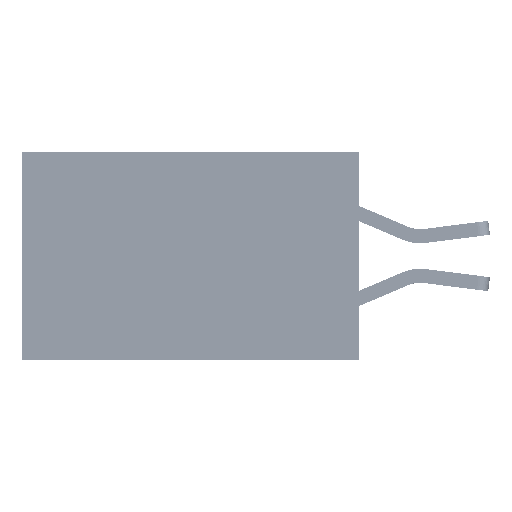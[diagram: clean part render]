
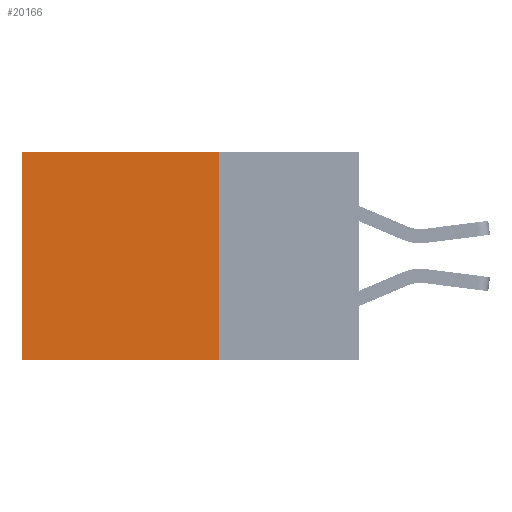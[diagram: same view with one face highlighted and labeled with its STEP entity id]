
A CAD part, left-side view. The second image highlights one B-rep face of the part: STEP entity #20166.
In plain terms, the highlighted planar face has unit normal (-1, 0, 0).
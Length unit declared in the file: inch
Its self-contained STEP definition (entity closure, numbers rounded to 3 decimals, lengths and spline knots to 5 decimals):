
#2309 = VERTEX_POINT ( 'NONE', #5757 ) ;
#3283 = LINE ( 'NONE', #34943, #49640 ) ;
#4492 = ORIENTED_EDGE ( 'NONE', *, *, #4638, .F. ) ;
#4638 = EDGE_CURVE ( 'NONE', #2309, #25689, #22918, .T. ) ;
#5257 = AXIS2_PLACEMENT_3D ( 'NONE', #21959, #42446, #38187 ) ;
#5658 = CARTESIAN_POINT ( 'NONE',  ( 0.2875, 0.25, 0. ) ) ;
#5757 = CARTESIAN_POINT ( 'NONE',  ( 0.2875, 0.25, -0.37 ) ) ;
#7684 = ORIENTED_EDGE ( 'NONE', *, *, #36085, .F. ) ;
#9734 = VERTEX_POINT ( 'NONE', #26997 ) ;
#10245 = FACE_OUTER_BOUND ( 'NONE', #40354, .T. ) ;
#11715 = ORIENTED_EDGE ( 'NONE', *, *, #41673, .T. ) ;
#14163 = LINE ( 'NONE', #5658, #38244 ) ;
#14734 = DIRECTION ( 'NONE',  ( 0., 0., -1. ) ) ;
#14960 = DIRECTION ( 'NONE',  ( 0., 1., 0. ) ) ;
#17117 = ORIENTED_EDGE ( 'NONE', *, *, #21518, .T. ) ;
#19547 = CARTESIAN_POINT ( 'NONE',  ( 0.2875, 0.6, -0.37 ) ) ;
#20166 = ADVANCED_FACE ( 'NONE', ( #10245 ), #47258, .F. ) ;
#21518 = EDGE_CURVE ( 'NONE', #37601, #9734, #42994, .T. ) ;
#21959 = CARTESIAN_POINT ( 'NONE',  ( 0.2875, 0.25, 0. ) ) ;
#22918 = LINE ( 'NONE', #31164, #44314 ) ;
#25689 = VERTEX_POINT ( 'NONE', #19547 ) ;
#26997 = CARTESIAN_POINT ( 'NONE',  ( 0.2875, 0.6, 0. ) ) ;
#27431 = VECTOR ( 'NONE', #50477, 39.37008 ) ;
#31164 = CARTESIAN_POINT ( 'NONE',  ( 0.2875, 0.25, -0.37 ) ) ;
#34202 = CARTESIAN_POINT ( 'NONE',  ( 0.2875, 0.25, 0. ) ) ;
#34943 = CARTESIAN_POINT ( 'NONE',  ( 0.2875, 0.6, 0. ) ) ;
#36085 = EDGE_CURVE ( 'NONE', #37601, #2309, #14163, .T. ) ;
#37601 = VERTEX_POINT ( 'NONE', #40502 ) ;
#38187 = DIRECTION ( 'NONE',  ( 0., 0., -1. ) ) ;
#38244 = VECTOR ( 'NONE', #50377, 39.37008 ) ;
#40354 = EDGE_LOOP ( 'NONE', ( #11715, #4492, #7684, #17117 ) ) ;
#40502 = CARTESIAN_POINT ( 'NONE',  ( 0.2875, 0.25, 0. ) ) ;
#41673 = EDGE_CURVE ( 'NONE', #9734, #25689, #3283, .T. ) ;
#42446 = DIRECTION ( 'NONE',  ( 1., 0., 0. ) ) ;
#42994 = LINE ( 'NONE', #34202, #27431 ) ;
#44314 = VECTOR ( 'NONE', #14960, 39.37008 ) ;
#47258 = PLANE ( 'NONE',  #5257 ) ;
#49640 = VECTOR ( 'NONE', #14734, 39.37008 ) ;
#50377 = DIRECTION ( 'NONE',  ( 0., 0., -1. ) ) ;
#50477 = DIRECTION ( 'NONE',  ( 0., 1., 0. ) ) ;
